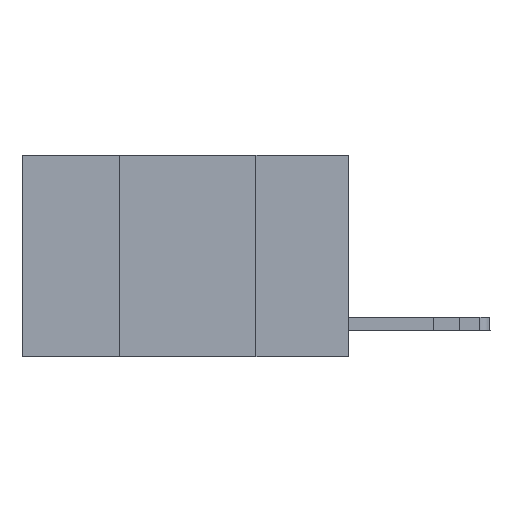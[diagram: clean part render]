
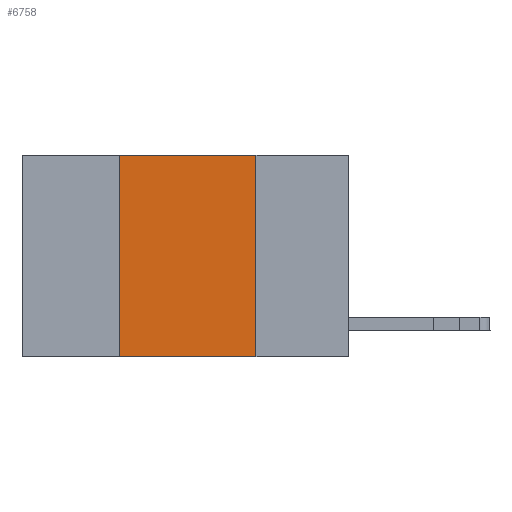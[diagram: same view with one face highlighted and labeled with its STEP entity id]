
A CAD part, left-side view. The second image highlights one B-rep face of the part: STEP entity #6758.
In plain terms, the highlighted planar face has unit normal (-1, 0, 0).
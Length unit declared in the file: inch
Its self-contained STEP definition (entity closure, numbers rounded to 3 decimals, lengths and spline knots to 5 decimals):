
#195 = CARTESIAN_POINT ( 'NONE',  ( 0., 0.17, 0. ) ) ;
#914 = VERTEX_POINT ( 'NONE', #195 ) ;
#976 = CARTESIAN_POINT ( 'NONE',  ( 0., 0.42, 0. ) ) ;
#2060 = DIRECTION ( 'NONE',  ( 0., 0., 1. ) ) ;
#2812 = ORIENTED_EDGE ( 'NONE', *, *, #9173, .T. ) ;
#3044 = CARTESIAN_POINT ( 'NONE',  ( 0., 0.42, -0.37 ) ) ;
#3231 = ORIENTED_EDGE ( 'NONE', *, *, #11465, .F. ) ;
#3627 = VERTEX_POINT ( 'NONE', #976 ) ;
#3857 = CARTESIAN_POINT ( 'NONE',  ( 0., 0.17, 0. ) ) ;
#4123 = LINE ( 'NONE', #5009, #12987 ) ;
#4325 = LINE ( 'NONE', #5471, #10531 ) ;
#4349 = CARTESIAN_POINT ( 'NONE',  ( 0., 0.6, 0. ) ) ;
#5009 = CARTESIAN_POINT ( 'NONE',  ( 0., 0.6, 0. ) ) ;
#5471 = CARTESIAN_POINT ( 'NONE',  ( 0., 0.6, -0.37 ) ) ;
#5522 = LINE ( 'NONE', #11328, #11325 ) ;
#5660 = VECTOR ( 'NONE', #7416, 39.37008 ) ;
#6181 = DIRECTION ( 'NONE',  ( 0., -1., 0. ) ) ;
#6693 = PLANE ( 'NONE',  #11382 ) ;
#6758 = ADVANCED_FACE ( 'NONE', ( #7893 ), #6693, .F. ) ;
#7416 = DIRECTION ( 'NONE',  ( 0., 0., -1. ) ) ;
#7893 = FACE_OUTER_BOUND ( 'NONE', #13958, .T. ) ;
#7913 = DIRECTION ( 'NONE',  ( 0., 0., -1. ) ) ;
#8781 = LINE ( 'NONE', #3857, #5660 ) ;
#8904 = VERTEX_POINT ( 'NONE', #10814 ) ;
#9173 = EDGE_CURVE ( 'NONE', #14662, #8904, #4325, .T. ) ;
#9942 = EDGE_CURVE ( 'NONE', #14662, #3627, #5522, .T. ) ;
#10531 = VECTOR ( 'NONE', #14564, 39.37008 ) ;
#10814 = CARTESIAN_POINT ( 'NONE',  ( 0., 0.17, -0.37 ) ) ;
#11325 = VECTOR ( 'NONE', #2060, 39.37008 ) ;
#11328 = CARTESIAN_POINT ( 'NONE',  ( 0., 0.42, 0. ) ) ;
#11382 = AXIS2_PLACEMENT_3D ( 'NONE', #4349, #14680, #7913 ) ;
#11465 = EDGE_CURVE ( 'NONE', #914, #8904, #8781, .T. ) ;
#12824 = ORIENTED_EDGE ( 'NONE', *, *, #9942, .F. ) ;
#12987 = VECTOR ( 'NONE', #6181, 39.37008 ) ;
#13666 = ORIENTED_EDGE ( 'NONE', *, *, #13887, .F. ) ;
#13887 = EDGE_CURVE ( 'NONE', #3627, #914, #4123, .T. ) ;
#13958 = EDGE_LOOP ( 'NONE', ( #3231, #13666, #12824, #2812 ) ) ;
#14564 = DIRECTION ( 'NONE',  ( 0., -1., 0. ) ) ;
#14662 = VERTEX_POINT ( 'NONE', #3044 ) ;
#14680 = DIRECTION ( 'NONE',  ( 1., 0., 0. ) ) ;
